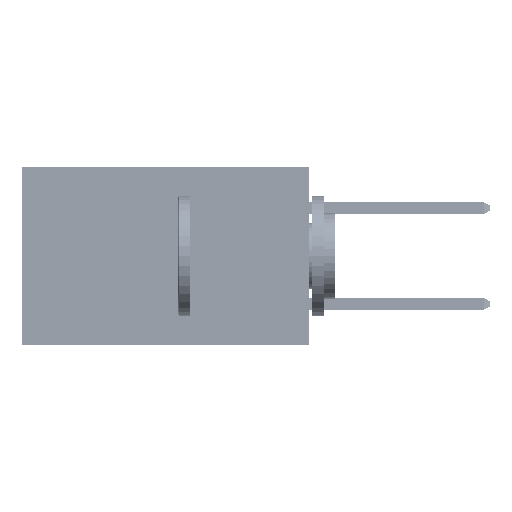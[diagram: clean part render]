
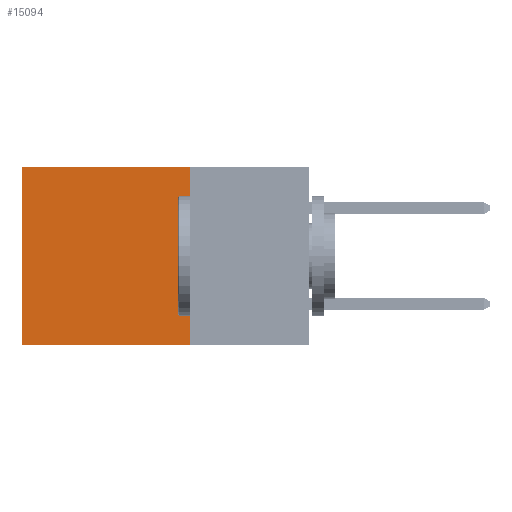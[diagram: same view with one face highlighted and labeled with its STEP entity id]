
A CAD part, left-side view. The second image highlights one B-rep face of the part: STEP entity #15094.
In plain terms, the highlighted planar face has unit normal (-1, 0, 0).
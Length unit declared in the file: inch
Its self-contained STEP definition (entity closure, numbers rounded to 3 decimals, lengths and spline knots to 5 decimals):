
#752 = CARTESIAN_POINT ( 'NONE',  ( 0.2875, 0.25, 0. ) ) ;
#2166 = CARTESIAN_POINT ( 'NONE',  ( 0.2875, 0.25, 0. ) ) ;
#4445 = LINE ( 'NONE', #25989, #28565 ) ;
#6243 = CARTESIAN_POINT ( 'NONE',  ( 0.2875, 0.6, 0. ) ) ;
#10019 = DIRECTION ( 'NONE',  ( 0., 1., 0. ) ) ;
#11540 = DIRECTION ( 'NONE',  ( 0., 0., -1. ) ) ;
#12962 = LINE ( 'NONE', #14067, #20796 ) ;
#13479 = DIRECTION ( 'NONE',  ( 0., 0., -1. ) ) ;
#14067 = CARTESIAN_POINT ( 'NONE',  ( 0.2875, 0.6, 0. ) ) ;
#14380 = EDGE_CURVE ( 'NONE', #21206, #41616, #4445, .T. ) ;
#15094 = ADVANCED_FACE ( 'NONE', ( #22491 ), #25262, .F. ) ;
#16947 = VECTOR ( 'NONE', #22805, 39.37008 ) ;
#19491 = CARTESIAN_POINT ( 'NONE',  ( 0.2875, 0.25, 0. ) ) ;
#20696 = EDGE_LOOP ( 'NONE', ( #33516, #37305, #29286, #45175 ) ) ;
#20796 = VECTOR ( 'NONE', #11540, 39.37008 ) ;
#21206 = VERTEX_POINT ( 'NONE', #19491 ) ;
#22491 = FACE_OUTER_BOUND ( 'NONE', #20696, .T. ) ;
#22805 = DIRECTION ( 'NONE',  ( 0., 1., 0. ) ) ;
#25262 = PLANE ( 'NONE',  #25661 ) ;
#25661 = AXIS2_PLACEMENT_3D ( 'NONE', #2166, #29152, #13479 ) ;
#25989 = CARTESIAN_POINT ( 'NONE',  ( 0.2875, 0.25, 0. ) ) ;
#26013 = EDGE_CURVE ( 'NONE', #21206, #38742, #43649, .T. ) ;
#27415 = CARTESIAN_POINT ( 'NONE',  ( 0.2875, 0.25, -0.37 ) ) ;
#27719 = DIRECTION ( 'NONE',  ( 0., 0., -1. ) ) ;
#27972 = CARTESIAN_POINT ( 'NONE',  ( 0.2875, 0.6, -0.37 ) ) ;
#28565 = VECTOR ( 'NONE', #10019, 39.37008 ) ;
#28971 = LINE ( 'NONE', #30040, #16947 ) ;
#29152 = DIRECTION ( 'NONE',  ( 1., 0., 0. ) ) ;
#29286 = ORIENTED_EDGE ( 'NONE', *, *, #26013, .F. ) ;
#30040 = CARTESIAN_POINT ( 'NONE',  ( 0.2875, 0.25, -0.37 ) ) ;
#30212 = EDGE_CURVE ( 'NONE', #38742, #36705, #28971, .T. ) ;
#33516 = ORIENTED_EDGE ( 'NONE', *, *, #37704, .T. ) ;
#36705 = VERTEX_POINT ( 'NONE', #27972 ) ;
#37305 = ORIENTED_EDGE ( 'NONE', *, *, #30212, .F. ) ;
#37704 = EDGE_CURVE ( 'NONE', #41616, #36705, #12962, .T. ) ;
#38742 = VERTEX_POINT ( 'NONE', #27415 ) ;
#41616 = VERTEX_POINT ( 'NONE', #6243 ) ;
#43649 = LINE ( 'NONE', #752, #45444 ) ;
#45175 = ORIENTED_EDGE ( 'NONE', *, *, #14380, .T. ) ;
#45444 = VECTOR ( 'NONE', #27719, 39.37008 ) ;
